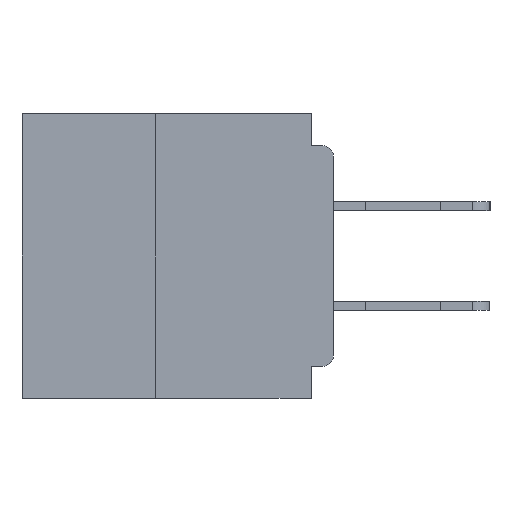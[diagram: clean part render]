
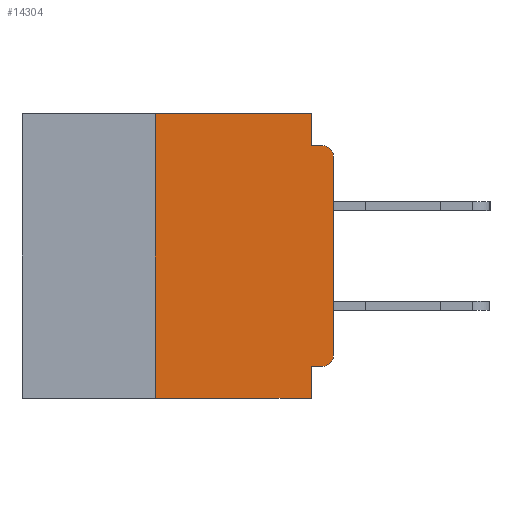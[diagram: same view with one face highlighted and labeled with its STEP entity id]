
A CAD part, left-side view. The second image highlights one B-rep face of the part: STEP entity #14304.
In plain terms, the highlighted planar face has unit normal (-1, 0, 0).
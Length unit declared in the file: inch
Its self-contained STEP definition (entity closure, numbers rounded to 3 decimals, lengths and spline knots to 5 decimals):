
#629 = VECTOR ( 'NONE', #28592, 39.37008 ) ;
#1401 = ORIENTED_EDGE ( 'NONE', *, *, #1682, .F. ) ;
#1682 = EDGE_CURVE ( 'NONE', #6489, #28140, #2578, .T. ) ;
#1987 = EDGE_CURVE ( 'NONE', #16996, #6489, #38378, .T. ) ;
#2133 = EDGE_CURVE ( 'NONE', #16342, #17562, #41362, .T. ) ;
#2578 = LINE ( 'NONE', #14912, #22227 ) ;
#3080 = EDGE_CURVE ( 'NONE', #44267, #17562, #27467, .T. ) ;
#4573 = CARTESIAN_POINT ( 'NONE',  ( 0., 0.015, -0.045 ) ) ;
#6489 = VERTEX_POINT ( 'NONE', #25996 ) ;
#7253 = EDGE_CURVE ( 'NONE', #28140, #16342, #45425, .T. ) ;
#7326 = DIRECTION ( 'NONE',  ( 0., 0., -1. ) ) ;
#9013 = CARTESIAN_POINT ( 'NONE',  ( 0., 0., -0.355 ) ) ;
#9636 = ORIENTED_EDGE ( 'NONE', *, *, #48183, .T. ) ;
#10686 = DIRECTION ( 'NONE',  ( -1., 0., 0. ) ) ;
#11109 = CARTESIAN_POINT ( 'NONE',  ( 0., 0.437, -0.4 ) ) ;
#11233 = LINE ( 'NONE', #43138, #40860 ) ;
#11360 = CARTESIAN_POINT ( 'NONE',  ( 0., 0.437, 0. ) ) ;
#11627 = ORIENTED_EDGE ( 'NONE', *, *, #7253, .F. ) ;
#12166 = LINE ( 'NONE', #11109, #41764 ) ;
#12727 = VERTEX_POINT ( 'NONE', #36584 ) ;
#13864 = ORIENTED_EDGE ( 'NONE', *, *, #1987, .F. ) ;
#14304 = ADVANCED_FACE ( 'NONE', ( #14696 ), #34597, .F. ) ;
#14696 = FACE_OUTER_BOUND ( 'NONE', #31400, .T. ) ;
#14863 = CARTESIAN_POINT ( 'NONE',  ( 0., 0.25, -0.4 ) ) ;
#14912 = CARTESIAN_POINT ( 'NONE',  ( 0., 0.437, 0. ) ) ;
#15278 = DIRECTION ( 'NONE',  ( 1., 0., 0. ) ) ;
#15884 = VECTOR ( 'NONE', #7326, 39.37008 ) ;
#16044 = CARTESIAN_POINT ( 'NONE',  ( 0., 0.031, 0. ) ) ;
#16190 = DIRECTION ( 'NONE',  ( 0., 0., -1. ) ) ;
#16342 = VERTEX_POINT ( 'NONE', #50007 ) ;
#16638 = DIRECTION ( 'NONE',  ( 0., 0., 1. ) ) ;
#16996 = VERTEX_POINT ( 'NONE', #50109 ) ;
#17562 = VERTEX_POINT ( 'NONE', #4573 ) ;
#17907 = VECTOR ( 'NONE', #16638, 39.37008 ) ;
#18307 = DIRECTION ( 'NONE',  ( 0., 0., -1. ) ) ;
#18469 = DIRECTION ( 'NONE',  ( -1., 0., 0. ) ) ;
#18479 = CARTESIAN_POINT ( 'NONE',  ( 0., 0.015, -0.06 ) ) ;
#18648 = ORIENTED_EDGE ( 'NONE', *, *, #24087, .F. ) ;
#18986 = DIRECTION ( 'NONE',  ( 0., -1., 0. ) ) ;
#20218 = VECTOR ( 'NONE', #33584, 39.37008 ) ;
#21514 = CARTESIAN_POINT ( 'NONE',  ( 0., 0., -0.34 ) ) ;
#22227 = VECTOR ( 'NONE', #48081, 39.37008 ) ;
#22661 = ORIENTED_EDGE ( 'NONE', *, *, #36836, .F. ) ;
#23029 = CARTESIAN_POINT ( 'NONE',  ( 0., 0.031, -0.4 ) ) ;
#24087 = EDGE_CURVE ( 'NONE', #12727, #35692, #26333, .T. ) ;
#24371 = CARTESIAN_POINT ( 'NONE',  ( 0., 0., -0.06 ) ) ;
#25996 = CARTESIAN_POINT ( 'NONE',  ( 0., 0.25, 0. ) ) ;
#26333 = LINE ( 'NONE', #9013, #629 ) ;
#26980 = AXIS2_PLACEMENT_3D ( 'NONE', #11360, #15278, #42258 ) ;
#27467 = CIRCLE ( 'NONE', #48764, 0.015 ) ;
#28140 = VERTEX_POINT ( 'NONE', #16044 ) ;
#28592 = DIRECTION ( 'NONE',  ( 0., 1., 0. ) ) ;
#29714 = CARTESIAN_POINT ( 'NONE',  ( 0., 0., 0. ) ) ;
#31212 = VECTOR ( 'NONE', #43277, 39.37008 ) ;
#31392 = CARTESIAN_POINT ( 'NONE',  ( 0., 0.031, -0.355 ) ) ;
#31400 = EDGE_LOOP ( 'NONE', ( #44747, #41079, #46808, #11627, #1401, #13864, #50072, #22661, #18648, #9636 ) ) ;
#31739 = LINE ( 'NONE', #29714, #20218 ) ;
#33584 = DIRECTION ( 'NONE',  ( 0., 0., 1. ) ) ;
#33953 = CARTESIAN_POINT ( 'NONE',  ( 0., 0.015, -0.34 ) ) ;
#34513 = CARTESIAN_POINT ( 'NONE',  ( 0., 0.031, 0. ) ) ;
#34597 = PLANE ( 'NONE',  #26980 ) ;
#35692 = VERTEX_POINT ( 'NONE', #31392 ) ;
#36584 = CARTESIAN_POINT ( 'NONE',  ( 0., 0.015, -0.355 ) ) ;
#36695 = VERTEX_POINT ( 'NONE', #23029 ) ;
#36836 = EDGE_CURVE ( 'NONE', #35692, #36695, #11233, .T. ) ;
#37745 = DIRECTION ( 'NONE',  ( 0., 0., -1. ) ) ;
#38378 = LINE ( 'NONE', #14863, #17907 ) ;
#38556 = EDGE_CURVE ( 'NONE', #47542, #44267, #31739, .T. ) ;
#39368 = EDGE_CURVE ( 'NONE', #16996, #36695, #12166, .T. ) ;
#40697 = CIRCLE ( 'NONE', #47978, 0.015 ) ;
#40860 = VECTOR ( 'NONE', #16190, 39.37008 ) ;
#41079 = ORIENTED_EDGE ( 'NONE', *, *, #3080, .T. ) ;
#41362 = LINE ( 'NONE', #47507, #31212 ) ;
#41764 = VECTOR ( 'NONE', #18986, 39.37008 ) ;
#42258 = DIRECTION ( 'NONE',  ( 0., 0., -1. ) ) ;
#43138 = CARTESIAN_POINT ( 'NONE',  ( 0., 0.031, -0.4 ) ) ;
#43277 = DIRECTION ( 'NONE',  ( 0., -1., 0. ) ) ;
#44267 = VERTEX_POINT ( 'NONE', #24371 ) ;
#44747 = ORIENTED_EDGE ( 'NONE', *, *, #38556, .T. ) ;
#45425 = LINE ( 'NONE', #34513, #15884 ) ;
#46808 = ORIENTED_EDGE ( 'NONE', *, *, #2133, .F. ) ;
#47507 = CARTESIAN_POINT ( 'NONE',  ( 0., 0., -0.045 ) ) ;
#47542 = VERTEX_POINT ( 'NONE', #21514 ) ;
#47978 = AXIS2_PLACEMENT_3D ( 'NONE', #33953, #10686, #37745 ) ;
#48081 = DIRECTION ( 'NONE',  ( 0., -1., 0. ) ) ;
#48183 = EDGE_CURVE ( 'NONE', #12727, #47542, #40697, .T. ) ;
#48764 = AXIS2_PLACEMENT_3D ( 'NONE', #18479, #18469, #18307 ) ;
#50007 = CARTESIAN_POINT ( 'NONE',  ( 0., 0.031, -0.045 ) ) ;
#50072 = ORIENTED_EDGE ( 'NONE', *, *, #39368, .T. ) ;
#50109 = CARTESIAN_POINT ( 'NONE',  ( 0., 0.25, -0.4 ) ) ;
